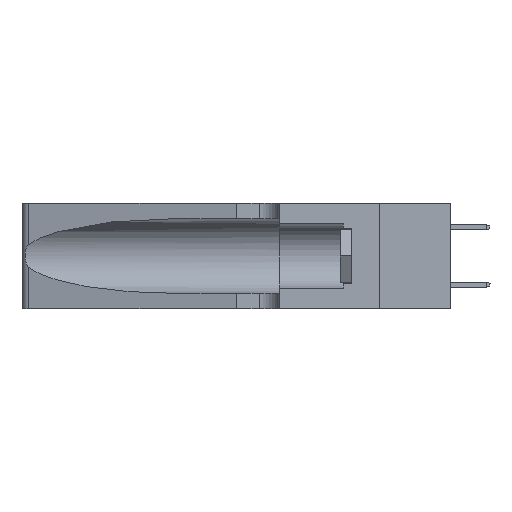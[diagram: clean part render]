
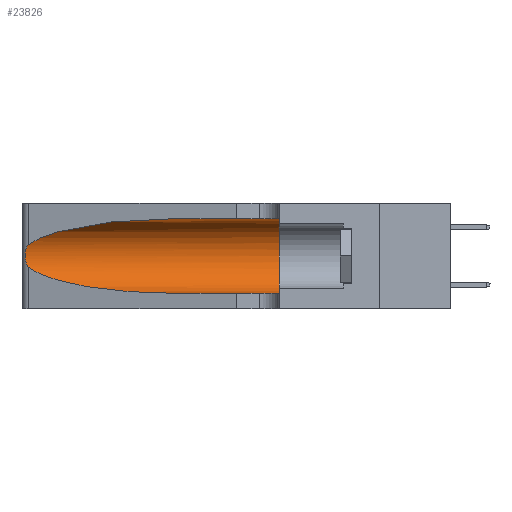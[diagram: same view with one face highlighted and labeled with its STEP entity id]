
A CAD part, left-side view. The second image highlights one B-rep face of the part: STEP entity #23826.
In plain terms, the highlighted cylindrical face has radius 3.308 mm (diameter 6.617 mm), a partial arc.
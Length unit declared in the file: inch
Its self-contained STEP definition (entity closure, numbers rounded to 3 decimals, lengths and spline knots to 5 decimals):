
#217 =( BOUNDED_CURVE ( )  B_SPLINE_CURVE ( 3, ( #22078, #28008, #38041, #34545 ),
 .UNSPECIFIED., .F., .T. ) 
 B_SPLINE_CURVE_WITH_KNOTS ( ( 4, 4 ),
 ( 1.5708, 2.84003 ),
 .UNSPECIFIED. ) 
 CURVE ( )  GEOMETRIC_REPRESENTATION_ITEM ( )  RATIONAL_B_SPLINE_CURVE ( ( 1., 0.87, 0.87, 1. ) ) 
 REPRESENTATION_ITEM ( '' )  );
#450 = CARTESIAN_POINT ( 'NONE',  ( 0.25856, 1.23593, 0.16098 ) ) ;
#1495 = EDGE_CURVE ( 'NONE', #23717, #38757, #39923, .T. ) ;
#2050 = CARTESIAN_POINT ( 'NONE',  ( 0.1305, 0.35, 0.31525 ) ) ;
#3162 = ORIENTED_EDGE ( 'NONE', *, *, #18694, .T. ) ;
#3315 = DIRECTION ( 'NONE',  ( 0., 0., -1. ) ) ;
#5512 = CARTESIAN_POINT ( 'NONE',  ( 0.1305, 0.72297, 0.05475 ) ) ;
#5718 = CARTESIAN_POINT ( 'NONE',  ( 0.25487, 1.22718, 0.14631 ) ) ;
#5954 = DIRECTION ( 'NONE',  ( 0., 0., 1. ) ) ;
#6170 = CARTESIAN_POINT ( 'NONE',  ( 0.26017, 1.23833, 0.17102 ) ) ;
#6178 = CARTESIAN_POINT ( 'NONE',  ( 0.25487, 1.22718, 0.22369 ) ) ;
#6320 = DIRECTION ( 'NONE',  ( 0., -1., 0. ) ) ;
#6577 = CARTESIAN_POINT ( 'NONE',  ( 0.25639, 1.23186, 0.15144 ) ) ;
#6706 = EDGE_CURVE ( 'NONE', #11439, #35303, #39268, .T. ) ;
#6990 = CARTESIAN_POINT ( 'NONE',  ( 0.25787, 1.23484, 0.2124 ) ) ;
#8222 = ORIENTED_EDGE ( 'NONE', *, *, #6706, .F. ) ;
#9028 = CARTESIAN_POINT ( 'NONE',  ( 0.1305, 0.35, 0.185 ) ) ;
#9197 = AXIS2_PLACEMENT_3D ( 'NONE', #9028, #24364, #5954 ) ;
#9449 = CARTESIAN_POINT ( 'NONE',  ( 0.25789, 1.23486, 0.15765 ) ) ;
#10012 = CARTESIAN_POINT ( 'NONE',  ( 0.1305, 1.61858, 0.31525 ) ) ;
#10064 = CARTESIAN_POINT ( 'NONE',  ( 0.25555, 1.22994, 0.2215 ) ) ;
#11439 = VERTEX_POINT ( 'NONE', #2050 ) ;
#12306 = CARTESIAN_POINT ( 'NONE',  ( 0.26075, 1.23896, 0.178 ) ) ;
#13323 = CARTESIAN_POINT ( 'NONE',  ( 0.1305, 1.61858, 0.185 ) ) ;
#14199 = LINE ( 'NONE', #26687, #22419 ) ;
#14912 = CARTESIAN_POINT ( 'NONE',  ( 0.2373, 1.15595, 0.08982 ) ) ;
#15369 = CARTESIAN_POINT ( 'NONE',  ( 0.26018, 1.23835, 0.19895 ) ) ;
#16991 = VECTOR ( 'NONE', #6320, 39.37008 ) ;
#18286 = EDGE_CURVE ( 'NONE', #38757, #34641, #36546, .T. ) ;
#18646 = CARTESIAN_POINT ( 'NONE',  ( 0.25555, 1.22993, 0.14849 ) ) ;
#18694 = EDGE_CURVE ( 'NONE', #38566, #23717, #217, .T. ) ;
#19466 = CARTESIAN_POINT ( 'NONE',  ( 0.1305, 0.35, 0.05475 ) ) ;
#21032 = ORIENTED_EDGE ( 'NONE', *, *, #18286, .T. ) ;
#22078 = CARTESIAN_POINT ( 'NONE',  ( 0.1305, 0.72297, 0.31525 ) ) ;
#22419 = VECTOR ( 'NONE', #36131, 39.37008 ) ;
#23617 = ORIENTED_EDGE ( 'NONE', *, *, #31760, .T. ) ;
#23717 = VERTEX_POINT ( 'NONE', #6178 ) ;
#23826 = ADVANCED_FACE ( 'NONE', ( #25813 ), #38119, .F. ) ;
#24364 = DIRECTION ( 'NONE',  ( 0., 1., 0. ) ) ;
#24642 = ORIENTED_EDGE ( 'NONE', *, *, #1495, .T. ) ;
#24666 = AXIS2_PLACEMENT_3D ( 'NONE', #13323, #28879, #3315 ) ;
#25524 = ORIENTED_EDGE ( 'NONE', *, *, #27107, .F. ) ;
#25702 = CARTESIAN_POINT ( 'NONE',  ( 0.1305, 0.72297, 0.05475 ) ) ;
#25813 = FACE_OUTER_BOUND ( 'NONE', #29400, .T. ) ;
#26687 = CARTESIAN_POINT ( 'NONE',  ( 0.1305, 1.61858, 0.05475 ) ) ;
#27107 = EDGE_CURVE ( 'NONE', #38566, #11439, #34973, .T. ) ;
#28008 = CARTESIAN_POINT ( 'NONE',  ( 0.18966, 0.96281, 0.31525 ) ) ;
#28465 = CARTESIAN_POINT ( 'NONE',  ( 0.26075, 1.23896, 0.19203 ) ) ;
#28879 = DIRECTION ( 'NONE',  ( 0., -1., 0. ) ) ;
#29400 = EDGE_LOOP ( 'NONE', ( #3162, #24642, #21032, #23617, #8222, #25524 ) ) ;
#31760 = EDGE_CURVE ( 'NONE', #34641, #35303, #14199, .T. ) ;
#31936 = CARTESIAN_POINT ( 'NONE',  ( 0.25854, 1.2359, 0.20912 ) ) ;
#33558 = CARTESIAN_POINT ( 'NONE',  ( 0.18966, 0.96281, 0.05475 ) ) ;
#34545 = CARTESIAN_POINT ( 'NONE',  ( 0.25487, 1.22718, 0.22369 ) ) ;
#34613 = CARTESIAN_POINT ( 'NONE',  ( 0.25487, 1.22718, 0.22369 ) ) ;
#34636 = CARTESIAN_POINT ( 'NONE',  ( 0.1305, 0.72297, 0.31525 ) ) ;
#34641 = VERTEX_POINT ( 'NONE', #25702 ) ;
#34973 = LINE ( 'NONE', #10012, #16991 ) ;
#35038 = CARTESIAN_POINT ( 'NONE',  ( 0.25639, 1.23184, 0.21858 ) ) ;
#35303 = VERTEX_POINT ( 'NONE', #19466 ) ;
#36131 = DIRECTION ( 'NONE',  ( 0., -1., 0. ) ) ;
#36207 = CARTESIAN_POINT ( 'NONE',  ( 0.25487, 1.22718, 0.14631 ) ) ;
#36546 =( BOUNDED_CURVE ( )  B_SPLINE_CURVE ( 3, ( #5718, #14912, #33558, #5512 ),
 .UNSPECIFIED., .F., .T. ) 
 B_SPLINE_CURVE_WITH_KNOTS ( ( 4, 4 ),
 ( 3.44316, 4.71239 ),
 .UNSPECIFIED. ) 
 CURVE ( )  GEOMETRIC_REPRESENTATION_ITEM ( )  RATIONAL_B_SPLINE_CURVE ( ( 1., 0.87, 0.87, 1. ) ) 
 REPRESENTATION_ITEM ( '' )  );
#37295 = CARTESIAN_POINT ( 'NONE',  ( 0.25487, 1.22718, 0.14631 ) ) ;
#38041 = CARTESIAN_POINT ( 'NONE',  ( 0.2373, 1.15595, 0.28018 ) ) ;
#38119 = CYLINDRICAL_SURFACE ( 'NONE', #24666, 0.13025 ) ;
#38566 = VERTEX_POINT ( 'NONE', #34636 ) ;
#38757 = VERTEX_POINT ( 'NONE', #36207 ) ;
#39268 = CIRCLE ( 'NONE', #9197, 0.13025 ) ;
#39923 = B_SPLINE_CURVE_WITH_KNOTS ( 'NONE', 3,
 ( #34613, #10064, #35038, #6990, #31936, #15369, #28465, #12306, #6170, #450, #9449, #6577, #18646, #37295 ),
 .UNSPECIFIED., .F., .F.,
 ( 4, 2, 2, 2, 2, 2, 4 ),
 ( 0., 0.00027, 0.00053, 0.00107, 0.0016, 0.00187, 0.00214 ),
 .UNSPECIFIED. ) ;
